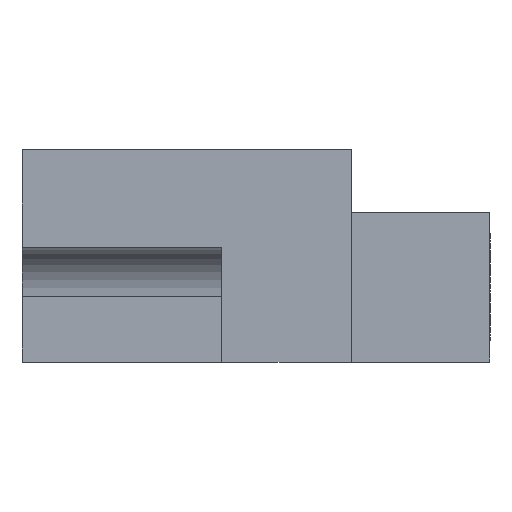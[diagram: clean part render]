
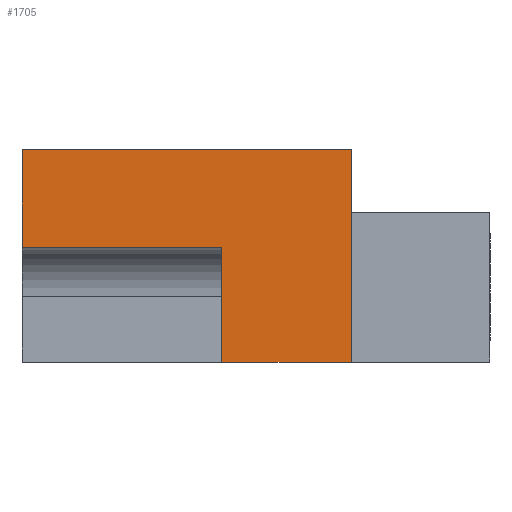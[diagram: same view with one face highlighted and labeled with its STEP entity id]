
A CAD part, left-side view. The second image highlights one B-rep face of the part: STEP entity #1705.
In plain terms, the highlighted planar face has unit normal (-1, 0, 0).
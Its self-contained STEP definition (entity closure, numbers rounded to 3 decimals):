
#216 = CARTESIAN_POINT ( 'NONE',  ( 0., 8.255, -13.487 ) ) ;
#335 = VERTEX_POINT ( 'NONE', #41493 ) ;
#418 = ORIENTED_EDGE ( 'NONE', *, *, #14918, .F. ) ;
#1005 = DIRECTION ( 'NONE',  ( 1., 0., 0. ) ) ;
#1705 = ADVANCED_FACE ( 'NONE', ( #2202 ), #4577, .F. ) ;
#1947 = ORIENTED_EDGE ( 'NONE', *, *, #13890, .F. ) ;
#2185 = CARTESIAN_POINT ( 'NONE',  ( 0., 20.955, -13.487 ) ) ;
#2202 = FACE_OUTER_BOUND ( 'NONE', #6591, .T. ) ;
#2911 = VECTOR ( 'NONE', #24968, 1000. ) ;
#3417 = LINE ( 'NONE', #2185, #2911 ) ;
#3972 = DIRECTION ( 'NONE',  ( 0., 1., 0. ) ) ;
#4577 = PLANE ( 'NONE',  #16728 ) ;
#5621 = CARTESIAN_POINT ( 'NONE',  ( 0., 8.255, -6.172 ) ) ;
#6007 = VECTOR ( 'NONE', #17370, 1000. ) ;
#6591 = EDGE_LOOP ( 'NONE', ( #33092, #25681, #12099, #418, #1947, #34490 ) ) ;
#6775 = DIRECTION ( 'NONE',  ( 0., 0., 1. ) ) ;
#7075 = LINE ( 'NONE', #14534, #32110 ) ;
#8861 = EDGE_CURVE ( 'NONE', #335, #36821, #32287, .T. ) ;
#10020 = CARTESIAN_POINT ( 'NONE',  ( 0., 0., 0. ) ) ;
#10556 = CARTESIAN_POINT ( 'NONE',  ( 0., 0., 0. ) ) ;
#12099 = ORIENTED_EDGE ( 'NONE', *, *, #8861, .F. ) ;
#13028 = VECTOR ( 'NONE', #6775, 1000. ) ;
#13404 = CARTESIAN_POINT ( 'NONE',  ( 0., -8.814, -13.487 ) ) ;
#13890 = EDGE_CURVE ( 'NONE', #35853, #38884, #7075, .T. ) ;
#14227 = DIRECTION ( 'NONE',  ( 0., -1., 0. ) ) ;
#14534 = CARTESIAN_POINT ( 'NONE',  ( 0., 8.255, -6.172 ) ) ;
#14766 = CARTESIAN_POINT ( 'NONE',  ( 0., 8.255, -13.487 ) ) ;
#14918 = EDGE_CURVE ( 'NONE', #38884, #335, #3417, .T. ) ;
#16075 = VERTEX_POINT ( 'NONE', #14766 ) ;
#16280 = EDGE_CURVE ( 'NONE', #16075, #35853, #35544, .T. ) ;
#16728 = AXIS2_PLACEMENT_3D ( 'NONE', #10020, #1005, #23807 ) ;
#17370 = DIRECTION ( 'NONE',  ( 0., 0., -1. ) ) ;
#19482 = CARTESIAN_POINT ( 'NONE',  ( 0., 20.955, -6.172 ) ) ;
#22520 = VECTOR ( 'NONE', #14227, 1000. ) ;
#23807 = DIRECTION ( 'NONE',  ( 0., 0., -1. ) ) ;
#24345 = DIRECTION ( 'NONE',  ( 0., 1., 0. ) ) ;
#24968 = DIRECTION ( 'NONE',  ( 0., 0., 1. ) ) ;
#25681 = ORIENTED_EDGE ( 'NONE', *, *, #32962, .F. ) ;
#26533 = VERTEX_POINT ( 'NONE', #34886 ) ;
#30932 = VECTOR ( 'NONE', #3972, 1000. ) ;
#31534 = CARTESIAN_POINT ( 'NONE',  ( 0., 0., 0. ) ) ;
#32110 = VECTOR ( 'NONE', #24345, 1000. ) ;
#32287 = LINE ( 'NONE', #33424, #22520 ) ;
#32962 = EDGE_CURVE ( 'NONE', #36821, #26533, #33116, .T. ) ;
#33092 = ORIENTED_EDGE ( 'NONE', *, *, #39985, .F. ) ;
#33116 = LINE ( 'NONE', #10556, #6007 ) ;
#33424 = CARTESIAN_POINT ( 'NONE',  ( 0., 11.506, 0. ) ) ;
#34490 = ORIENTED_EDGE ( 'NONE', *, *, #16280, .F. ) ;
#34886 = CARTESIAN_POINT ( 'NONE',  ( 0., 0., -13.487 ) ) ;
#35544 = LINE ( 'NONE', #216, #13028 ) ;
#35853 = VERTEX_POINT ( 'NONE', #5621 ) ;
#36821 = VERTEX_POINT ( 'NONE', #31534 ) ;
#38572 = LINE ( 'NONE', #13404, #30932 ) ;
#38884 = VERTEX_POINT ( 'NONE', #19482 ) ;
#39985 = EDGE_CURVE ( 'NONE', #26533, #16075, #38572, .T. ) ;
#41493 = CARTESIAN_POINT ( 'NONE',  ( 0., 20.955, 0. ) ) ;
